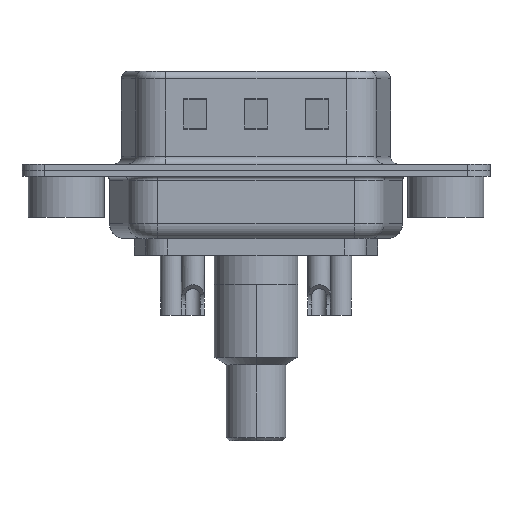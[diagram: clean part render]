
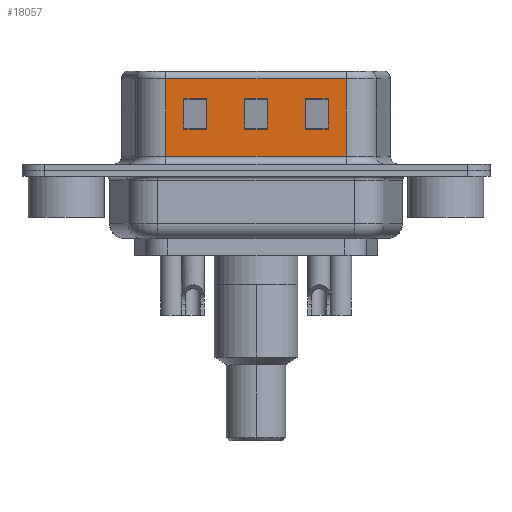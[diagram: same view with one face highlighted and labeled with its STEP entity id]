
A CAD part, front view. The second image highlights one B-rep face of the part: STEP entity #18057.
In plain terms, the highlighted planar face has unit normal (0, -1, 0).
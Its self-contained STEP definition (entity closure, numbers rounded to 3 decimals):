
#64 = DIRECTION ( 'NONE',  ( 0., 0., -1. ) ) ;
#203 = VECTOR ( 'NONE', #12755, 1000. ) ;
#211 = CARTESIAN_POINT ( 'NONE',  ( 9.25, -4.58, 6.52 ) ) ;
#231 = VERTEX_POINT ( 'NONE', #20111 ) ;
#512 = VERTEX_POINT ( 'NONE', #15934 ) ;
#677 = DIRECTION ( 'NONE',  ( 0., 0., 1. ) ) ;
#814 = VERTEX_POINT ( 'NONE', #9646 ) ;
#921 = CARTESIAN_POINT ( 'NONE',  ( 22.45, -4.58, 2.705 ) ) ;
#1064 = CARTESIAN_POINT ( 'NONE',  ( 7.75, -4.58, 4.705 ) ) ;
#1392 = CARTESIAN_POINT ( 'NONE',  ( 11.75, -4.58, 6.52 ) ) ;
#1470 = VECTOR ( 'NONE', #64, 1000. ) ;
#1931 = VECTOR ( 'NONE', #17384, 1000. ) ;
#2113 = ORIENTED_EDGE ( 'NONE', *, *, #2614, .T. ) ;
#2246 = ORIENTED_EDGE ( 'NONE', *, *, #3297, .T. ) ;
#2345 = ORIENTED_EDGE ( 'NONE', *, *, #2898, .T. ) ;
#2485 = EDGE_LOOP ( 'NONE', ( #4627, #7541, #7087, #2113 ) ) ;
#2522 = EDGE_CURVE ( 'NONE', #11391, #6846, #3032, .T. ) ;
#2588 = EDGE_CURVE ( 'NONE', #10499, #12667, #10366, .T. ) ;
#2614 = EDGE_CURVE ( 'NONE', #12667, #8099, #18008, .T. ) ;
#2646 = EDGE_CURVE ( 'NONE', #7922, #10499, #14462, .T. ) ;
#2717 = EDGE_CURVE ( 'NONE', #8099, #7922, #12588, .T. ) ;
#2790 = ORIENTED_EDGE ( 'NONE', *, *, #3038, .T. ) ;
#2898 = EDGE_CURVE ( 'NONE', #5004, #13268, #9144, .T. ) ;
#2926 = EDGE_CURVE ( 'NONE', #10361, #11839, #4365, .T. ) ;
#2930 = VECTOR ( 'NONE', #8523, 1000. ) ;
#3014 = EDGE_CURVE ( 'NONE', #11839, #5004, #19462, .T. ) ;
#3032 = LINE ( 'NONE', #14288, #6705 ) ;
#3038 = EDGE_CURVE ( 'NONE', #13268, #10361, #18972, .T. ) ;
#3132 = EDGE_CURVE ( 'NONE', #3643, #231, #17989, .T. ) ;
#3229 = DIRECTION ( 'NONE',  ( 0., 0., -1. ) ) ;
#3266 = EDGE_CURVE ( 'NONE', #814, #3643, #15623, .T. ) ;
#3297 = EDGE_CURVE ( 'NONE', #3878, #814, #18714, .T. ) ;
#3465 = EDGE_CURVE ( 'NONE', #231, #3878, #12307, .T. ) ;
#3643 = VERTEX_POINT ( 'NONE', #1064 ) ;
#3671 = EDGE_CURVE ( 'NONE', #512, #11391, #19444, .T. ) ;
#3725 = EDGE_CURVE ( 'NONE', #9313, #512, #9359, .T. ) ;
#3878 = VERTEX_POINT ( 'NONE', #9773 ) ;
#4365 = LINE ( 'NONE', #921, #203 ) ;
#4584 = CARTESIAN_POINT ( 'NONE',  ( 6.55, -4.58, 6.52 ) ) ;
#4627 = ORIENTED_EDGE ( 'NONE', *, *, #2717, .T. ) ;
#4757 = EDGE_CURVE ( 'NONE', #9313, #6846, #9809, .T. ) ;
#5004 = VERTEX_POINT ( 'NONE', #14771 ) ;
#5035 = AXIS2_PLACEMENT_3D ( 'NONE', #11684, #10151, #677 ) ;
#6122 = VECTOR ( 'NONE', #14812, 1000. ) ;
#6436 = CARTESIAN_POINT ( 'NONE',  ( 18.45, -4.58, 0.9 ) ) ;
#6595 = VECTOR ( 'NONE', #3229, 1000. ) ;
#6705 = VECTOR ( 'NONE', #18742, 1000. ) ;
#6842 = VECTOR ( 'NONE', #16334, 1000. ) ;
#6846 = VERTEX_POINT ( 'NONE', #6436 ) ;
#7087 = ORIENTED_EDGE ( 'NONE', *, *, #2588, .T. ) ;
#7282 = EDGE_LOOP ( 'NONE', ( #13532, #2246, #16499, #12381 ) ) ;
#7541 = ORIENTED_EDGE ( 'NONE', *, *, #2646, .T. ) ;
#7818 = CARTESIAN_POINT ( 'NONE',  ( 7.75, -4.58, 6.52 ) ) ;
#7841 = DIRECTION ( 'NONE',  ( 1., 0., 0. ) ) ;
#7916 = DIRECTION ( 'NONE',  ( 0., 0., -1. ) ) ;
#7922 = VERTEX_POINT ( 'NONE', #13534 ) ;
#8095 = ORIENTED_EDGE ( 'NONE', *, *, #2926, .T. ) ;
#8099 = VERTEX_POINT ( 'NONE', #16161 ) ;
#8138 = DIRECTION ( 'NONE',  ( -1., 0., 0. ) ) ;
#8371 = CARTESIAN_POINT ( 'NONE',  ( 17.25, -4.58, 2.705 ) ) ;
#8523 = DIRECTION ( 'NONE',  ( 0., 0., 1. ) ) ;
#8582 = PLANE ( 'NONE',  #5035 ) ;
#8640 = VECTOR ( 'NONE', #17125, 1000. ) ;
#8708 = ORIENTED_EDGE ( 'NONE', *, *, #3014, .T. ) ;
#9002 = FACE_BOUND ( 'NONE', #7282, .T. ) ;
#9005 = ORIENTED_EDGE ( 'NONE', *, *, #4757, .F. ) ;
#9144 = LINE ( 'NONE', #11718, #8640 ) ;
#9313 = VERTEX_POINT ( 'NONE', #16630 ) ;
#9359 = LINE ( 'NONE', #14625, #16567 ) ;
#9381 = VECTOR ( 'NONE', #7841, 1000. ) ;
#9646 = CARTESIAN_POINT ( 'NONE',  ( 7.75, -4.58, 2.705 ) ) ;
#9682 = CARTESIAN_POINT ( 'NONE',  ( 17.25, -4.58, 4.705 ) ) ;
#9773 = CARTESIAN_POINT ( 'NONE',  ( 9.25, -4.58, 2.705 ) ) ;
#9809 = LINE ( 'NONE', #14418, #13445 ) ;
#10151 = DIRECTION ( 'NONE',  ( 0., 1., 0. ) ) ;
#10280 = ORIENTED_EDGE ( 'NONE', *, *, #3671, .T. ) ;
#10361 = VERTEX_POINT ( 'NONE', #8371 ) ;
#10366 = LINE ( 'NONE', #13058, #6122 ) ;
#10499 = VERTEX_POINT ( 'NONE', #18221 ) ;
#10552 = CARTESIAN_POINT ( 'NONE',  ( 17.25, -4.58, 6.52 ) ) ;
#11093 = VECTOR ( 'NONE', #15154, 1000. ) ;
#11391 = VERTEX_POINT ( 'NONE', #14153 ) ;
#11581 = CARTESIAN_POINT ( 'NONE',  ( 15.75, -4.58, 6.52 ) ) ;
#11684 = CARTESIAN_POINT ( 'NONE',  ( 18.45, -4.58, 6.52 ) ) ;
#11718 = CARTESIAN_POINT ( 'NONE',  ( 22.45, -4.58, 4.705 ) ) ;
#11839 = VERTEX_POINT ( 'NONE', #15320 ) ;
#11870 = EDGE_LOOP ( 'NONE', ( #9005, #14366, #10280, #14601 ) ) ;
#12307 = LINE ( 'NONE', #211, #13280 ) ;
#12381 = ORIENTED_EDGE ( 'NONE', *, *, #3132, .T. ) ;
#12588 = LINE ( 'NONE', #16002, #16603 ) ;
#12667 = VERTEX_POINT ( 'NONE', #19075 ) ;
#12755 = DIRECTION ( 'NONE',  ( -1., 0., 0. ) ) ;
#13058 = CARTESIAN_POINT ( 'NONE',  ( 18.45, -4.58, 2.705 ) ) ;
#13157 = FACE_OUTER_BOUND ( 'NONE', #11870, .T. ) ;
#13268 = VERTEX_POINT ( 'NONE', #9682 ) ;
#13280 = VECTOR ( 'NONE', #13964, 1000. ) ;
#13445 = VECTOR ( 'NONE', #7916, 1000. ) ;
#13532 = ORIENTED_EDGE ( 'NONE', *, *, #3465, .T. ) ;
#13534 = CARTESIAN_POINT ( 'NONE',  ( 13.25, -4.58, 4.705 ) ) ;
#13600 = FACE_BOUND ( 'NONE', #19784, .T. ) ;
#13964 = DIRECTION ( 'NONE',  ( 0., 0., -1. ) ) ;
#14153 = CARTESIAN_POINT ( 'NONE',  ( 6.55, -4.58, 0.9 ) ) ;
#14288 = CARTESIAN_POINT ( 'NONE',  ( 18.45, -4.58, 0.9 ) ) ;
#14366 = ORIENTED_EDGE ( 'NONE', *, *, #3725, .T. ) ;
#14418 = CARTESIAN_POINT ( 'NONE',  ( 18.45, -4.58, 6.52 ) ) ;
#14462 = LINE ( 'NONE', #14899, #1470 ) ;
#14601 = ORIENTED_EDGE ( 'NONE', *, *, #2522, .T. ) ;
#14625 = CARTESIAN_POINT ( 'NONE',  ( 18.45, -4.58, 6.02 ) ) ;
#14771 = CARTESIAN_POINT ( 'NONE',  ( 15.75, -4.58, 4.705 ) ) ;
#14812 = DIRECTION ( 'NONE',  ( -1., 0., 0. ) ) ;
#14899 = CARTESIAN_POINT ( 'NONE',  ( 13.25, -4.58, 6.52 ) ) ;
#15037 = CARTESIAN_POINT ( 'NONE',  ( 14.45, -4.58, 2.705 ) ) ;
#15154 = DIRECTION ( 'NONE',  ( 0., 0., 1. ) ) ;
#15320 = CARTESIAN_POINT ( 'NONE',  ( 15.75, -4.58, 2.705 ) ) ;
#15623 = LINE ( 'NONE', #7818, #11093 ) ;
#15934 = CARTESIAN_POINT ( 'NONE',  ( 6.55, -4.58, 6.02 ) ) ;
#16002 = CARTESIAN_POINT ( 'NONE',  ( 18.45, -4.58, 4.705 ) ) ;
#16161 = CARTESIAN_POINT ( 'NONE',  ( 11.75, -4.58, 4.705 ) ) ;
#16334 = DIRECTION ( 'NONE',  ( -1., 0., 0. ) ) ;
#16499 = ORIENTED_EDGE ( 'NONE', *, *, #3266, .T. ) ;
#16567 = VECTOR ( 'NONE', #8138, 1000. ) ;
#16603 = VECTOR ( 'NONE', #20132, 1000. ) ;
#16630 = CARTESIAN_POINT ( 'NONE',  ( 18.45, -4.58, 6.02 ) ) ;
#17125 = DIRECTION ( 'NONE',  ( 1., 0., 0. ) ) ;
#17145 = FACE_BOUND ( 'NONE', #2485, .T. ) ;
#17384 = DIRECTION ( 'NONE',  ( 0., 0., -1. ) ) ;
#17738 = CARTESIAN_POINT ( 'NONE',  ( 14.45, -4.58, 4.705 ) ) ;
#17989 = LINE ( 'NONE', #17738, #9381 ) ;
#18008 = LINE ( 'NONE', #1392, #18501 ) ;
#18057 = ADVANCED_FACE ( 'NONE', ( #9002, #13600, #17145, #13157 ), #8582, .F. ) ;
#18221 = CARTESIAN_POINT ( 'NONE',  ( 13.25, -4.58, 2.705 ) ) ;
#18501 = VECTOR ( 'NONE', #18767, 1000. ) ;
#18714 = LINE ( 'NONE', #15037, #6842 ) ;
#18742 = DIRECTION ( 'NONE',  ( 1., 0., 0. ) ) ;
#18767 = DIRECTION ( 'NONE',  ( 0., 0., 1. ) ) ;
#18972 = LINE ( 'NONE', #10552, #6595 ) ;
#19075 = CARTESIAN_POINT ( 'NONE',  ( 11.75, -4.58, 2.705 ) ) ;
#19444 = LINE ( 'NONE', #4584, #1931 ) ;
#19462 = LINE ( 'NONE', #11581, #2930 ) ;
#19784 = EDGE_LOOP ( 'NONE', ( #2790, #8095, #8708, #2345 ) ) ;
#20111 = CARTESIAN_POINT ( 'NONE',  ( 9.25, -4.58, 4.705 ) ) ;
#20132 = DIRECTION ( 'NONE',  ( 1., 0., 0. ) ) ;
